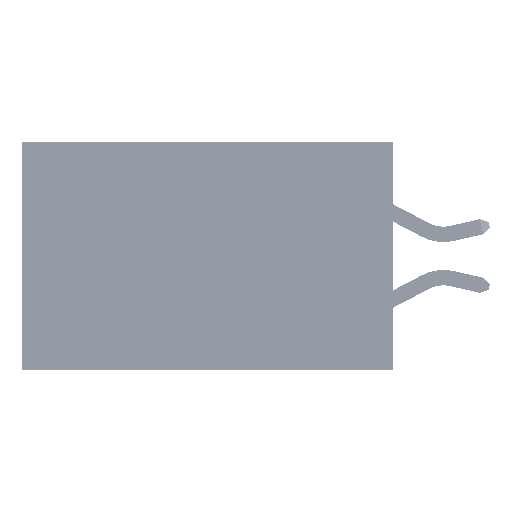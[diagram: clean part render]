
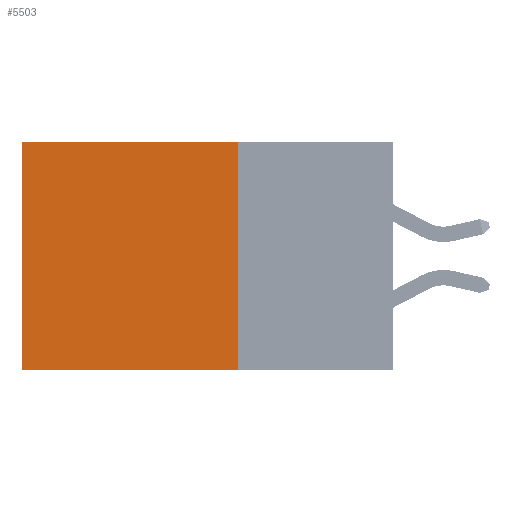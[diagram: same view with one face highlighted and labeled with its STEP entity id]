
A CAD part, left-side view. The second image highlights one B-rep face of the part: STEP entity #5503.
In plain terms, the highlighted planar face has unit normal (-1, 0, 0).
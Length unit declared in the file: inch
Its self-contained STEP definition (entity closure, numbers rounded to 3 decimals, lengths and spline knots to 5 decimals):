
#261 = VECTOR ( 'NONE', #7173, 39.37008 ) ;
#437 = FACE_OUTER_BOUND ( 'NONE', #455, .T. ) ;
#455 = EDGE_LOOP ( 'NONE', ( #568, #25909, #37877, #5237 ) ) ;
#568 = ORIENTED_EDGE ( 'NONE', *, *, #17802, .T. ) ;
#611 = DIRECTION ( 'NONE',  ( 0., 0., -1. ) ) ;
#1044 = VERTEX_POINT ( 'NONE', #43645 ) ;
#1463 = AXIS2_PLACEMENT_3D ( 'NONE', #32996, #11678, #26289 ) ;
#2514 = EDGE_CURVE ( 'NONE', #18757, #21779, #11402, .T. ) ;
#3904 = VECTOR ( 'NONE', #42581, 39.37008 ) ;
#5237 = ORIENTED_EDGE ( 'NONE', *, *, #22576, .T. ) ;
#5419 = CARTESIAN_POINT ( 'NONE',  ( 0.2875, 0.25, -0.37 ) ) ;
#5503 = ADVANCED_FACE ( 'NONE', ( #437 ), #15039, .F. ) ;
#7173 = DIRECTION ( 'NONE',  ( 0., 1., 0. ) ) ;
#8739 = CARTESIAN_POINT ( 'NONE',  ( 0.2875, 0.25, 0. ) ) ;
#11402 = LINE ( 'NONE', #8739, #13947 ) ;
#11678 = DIRECTION ( 'NONE',  ( 1., 0., 0. ) ) ;
#12566 = CARTESIAN_POINT ( 'NONE',  ( 0.2875, 0.25, -0.37 ) ) ;
#13947 = VECTOR ( 'NONE', #611, 39.37008 ) ;
#15039 = PLANE ( 'NONE',  #1463 ) ;
#16235 = LINE ( 'NONE', #27288, #3904 ) ;
#17802 = EDGE_CURVE ( 'NONE', #25941, #1044, #16235, .T. ) ;
#18252 = EDGE_CURVE ( 'NONE', #21779, #1044, #41323, .T. ) ;
#18757 = VERTEX_POINT ( 'NONE', #34085 ) ;
#21779 = VERTEX_POINT ( 'NONE', #12566 ) ;
#22576 = EDGE_CURVE ( 'NONE', #18757, #25941, #36591, .T. ) ;
#24099 = DIRECTION ( 'NONE',  ( 0., 1., 0. ) ) ;
#25370 = CARTESIAN_POINT ( 'NONE',  ( 0.2875, 0.25, 0. ) ) ;
#25909 = ORIENTED_EDGE ( 'NONE', *, *, #18252, .F. ) ;
#25941 = VERTEX_POINT ( 'NONE', #39164 ) ;
#26289 = DIRECTION ( 'NONE',  ( 0., 0., -1. ) ) ;
#27288 = CARTESIAN_POINT ( 'NONE',  ( 0.2875, 0.6, 0. ) ) ;
#32996 = CARTESIAN_POINT ( 'NONE',  ( 0.2875, 0.25, 0. ) ) ;
#34085 = CARTESIAN_POINT ( 'NONE',  ( 0.2875, 0.25, 0. ) ) ;
#36591 = LINE ( 'NONE', #25370, #261 ) ;
#37877 = ORIENTED_EDGE ( 'NONE', *, *, #2514, .F. ) ;
#39164 = CARTESIAN_POINT ( 'NONE',  ( 0.2875, 0.6, 0. ) ) ;
#41323 = LINE ( 'NONE', #5419, #43671 ) ;
#42581 = DIRECTION ( 'NONE',  ( 0., 0., -1. ) ) ;
#43645 = CARTESIAN_POINT ( 'NONE',  ( 0.2875, 0.6, -0.37 ) ) ;
#43671 = VECTOR ( 'NONE', #24099, 39.37008 ) ;
